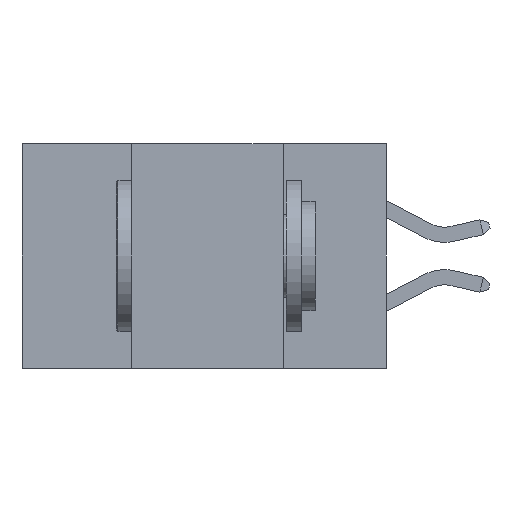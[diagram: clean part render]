
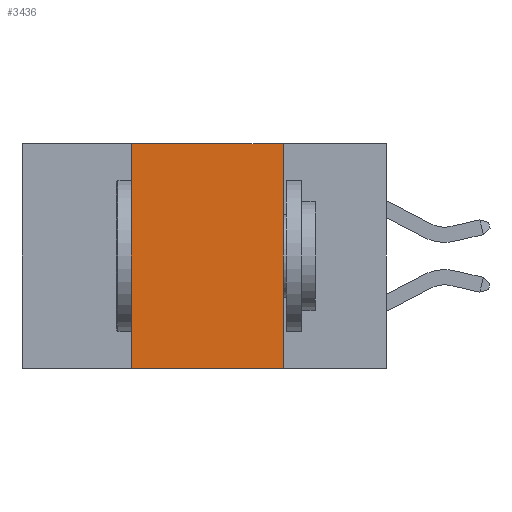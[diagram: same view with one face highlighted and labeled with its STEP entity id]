
A CAD part, left-side view. The second image highlights one B-rep face of the part: STEP entity #3436.
In plain terms, the highlighted planar face has unit normal (-1, 0, 0).
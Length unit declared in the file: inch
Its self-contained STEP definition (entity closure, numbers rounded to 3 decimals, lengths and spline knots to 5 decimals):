
#199 = CARTESIAN_POINT ( 'NONE',  ( 0., 0.17, 0. ) ) ;
#1053 = VERTEX_POINT ( 'NONE', #15897 ) ;
#2416 = AXIS2_PLACEMENT_3D ( 'NONE', #13674, #14033, #14013 ) ;
#2979 = EDGE_CURVE ( 'NONE', #1053, #3234, #13012, .T. ) ;
#3234 = VERTEX_POINT ( 'NONE', #21701 ) ;
#3436 = ADVANCED_FACE ( 'NONE', ( #17831 ), #13562, .F. ) ;
#5101 = VERTEX_POINT ( 'NONE', #199 ) ;
#5886 = EDGE_LOOP ( 'NONE', ( #20456, #13519, #10632, #12359 ) ) ;
#7946 = VECTOR ( 'NONE', #25457, 39.37008 ) ;
#8459 = EDGE_CURVE ( 'NONE', #1053, #25421, #24314, .T. ) ;
#9003 = LINE ( 'NONE', #24217, #15127 ) ;
#9103 = CARTESIAN_POINT ( 'NONE',  ( 0., 0.42, 0. ) ) ;
#9891 = DIRECTION ( 'NONE',  ( 0., -1., 0. ) ) ;
#10632 = ORIENTED_EDGE ( 'NONE', *, *, #8459, .F. ) ;
#12359 = ORIENTED_EDGE ( 'NONE', *, *, #2979, .T. ) ;
#13012 = LINE ( 'NONE', #22494, #23297 ) ;
#13460 = EDGE_CURVE ( 'NONE', #25421, #5101, #9003, .T. ) ;
#13519 = ORIENTED_EDGE ( 'NONE', *, *, #13460, .F. ) ;
#13562 = PLANE ( 'NONE',  #2416 ) ;
#13674 = CARTESIAN_POINT ( 'NONE',  ( 0., 0.6, 0. ) ) ;
#14013 = DIRECTION ( 'NONE',  ( 0., 0., -1. ) ) ;
#14033 = DIRECTION ( 'NONE',  ( 1., 0., 0. ) ) ;
#15127 = VECTOR ( 'NONE', #9891, 39.37008 ) ;
#15897 = CARTESIAN_POINT ( 'NONE',  ( 0., 0.42, -0.37 ) ) ;
#16078 = VECTOR ( 'NONE', #16920, 39.37008 ) ;
#16920 = DIRECTION ( 'NONE',  ( 0., 0., -1. ) ) ;
#17831 = FACE_OUTER_BOUND ( 'NONE', #5886, .T. ) ;
#19506 = EDGE_CURVE ( 'NONE', #5101, #3234, #21558, .T. ) ;
#20456 = ORIENTED_EDGE ( 'NONE', *, *, #19506, .F. ) ;
#21077 = CARTESIAN_POINT ( 'NONE',  ( 0., 0.17, 0. ) ) ;
#21558 = LINE ( 'NONE', #21077, #16078 ) ;
#21701 = CARTESIAN_POINT ( 'NONE',  ( 0., 0.17, -0.37 ) ) ;
#22189 = CARTESIAN_POINT ( 'NONE',  ( 0., 0.42, 0. ) ) ;
#22494 = CARTESIAN_POINT ( 'NONE',  ( 0., 0.6, -0.37 ) ) ;
#22616 = DIRECTION ( 'NONE',  ( 0., -1., 0. ) ) ;
#23297 = VECTOR ( 'NONE', #22616, 39.37008 ) ;
#24217 = CARTESIAN_POINT ( 'NONE',  ( 0., 0.6, 0. ) ) ;
#24314 = LINE ( 'NONE', #9103, #7946 ) ;
#25421 = VERTEX_POINT ( 'NONE', #22189 ) ;
#25457 = DIRECTION ( 'NONE',  ( 0., 0., 1. ) ) ;
